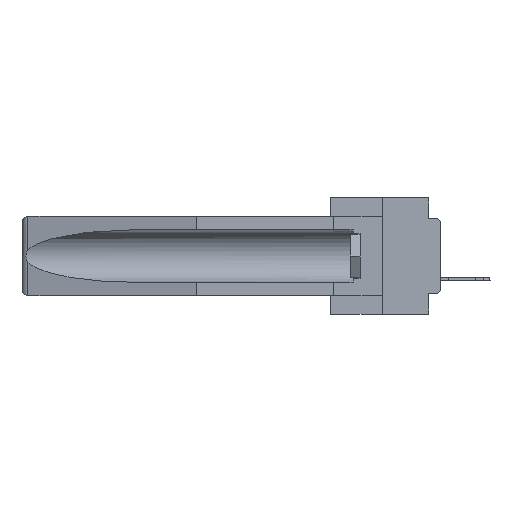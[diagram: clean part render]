
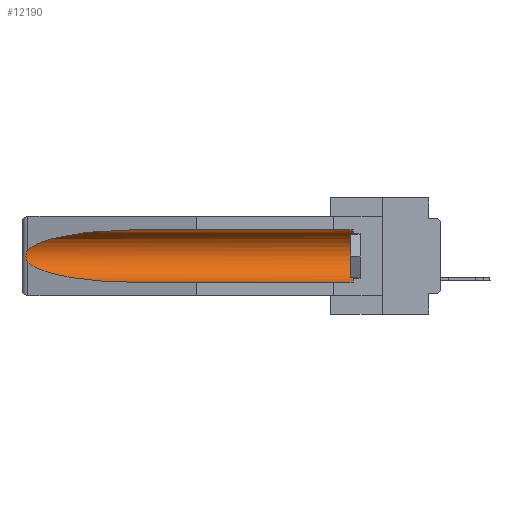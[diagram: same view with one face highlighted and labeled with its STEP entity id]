
A CAD part, left-side view. The second image highlights one B-rep face of the part: STEP entity #12190.
In plain terms, the highlighted cylindrical face has radius 2.857 mm (diameter 5.715 mm), a partial arc.
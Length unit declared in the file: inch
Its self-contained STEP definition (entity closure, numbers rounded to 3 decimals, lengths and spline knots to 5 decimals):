
#623 = CARTESIAN_POINT ( 'NONE',  ( 0.155, 1.07973, -0.059 ) ) ;
#852 = CARTESIAN_POINT ( 'NONE',  ( 0.26597, 1.5296, -0.19026 ) ) ;
#1108 = VERTEX_POINT ( 'NONE', #21107 ) ;
#1117 = EDGE_CURVE ( 'NONE', #18247, #1108, #5084, .T. ) ;
#1607 = DIRECTION ( 'NONE',  ( 0., 0., 1. ) ) ;
#1929 = CARTESIAN_POINT ( 'NONE',  ( 0.25451, 1.48313, -0.24835 ) ) ;
#3759 = ORIENTED_EDGE ( 'NONE', *, *, #10350, .T. ) ;
#4163 = CARTESIAN_POINT ( 'NONE',  ( 0.155, 1.07973, -0.284 ) ) ;
#5084 = CIRCLE ( 'NONE', #31580, 0.1125 ) ;
#5735 = VECTOR ( 'NONE', #5824, 39.37008 ) ;
#5824 = DIRECTION ( 'NONE',  ( 0., 1., 0. ) ) ;
#6933 = ORIENTED_EDGE ( 'NONE', *, *, #9786, .T. ) ;
#7885 = EDGE_CURVE ( 'NONE', #1108, #22006, #8084, .T. ) ;
#7907 = LINE ( 'NONE', #23471, #10756 ) ;
#7972 = EDGE_CURVE ( 'NONE', #18247, #27088, #7907, .T. ) ;
#8084 = LINE ( 'NONE', #13644, #5735 ) ;
#8950 = CARTESIAN_POINT ( 'NONE',  ( 0.26537, 1.52718, -0.19328 ) ) ;
#9365 = CARTESIAN_POINT ( 'NONE',  ( 0.21114, 1.30732, -0.284 ) ) ;
#9786 = EDGE_CURVE ( 'NONE', #22006, #15409, #31780, .T. ) ;
#9993 = VERTEX_POINT ( 'NONE', #33556 ) ;
#10173 = ORIENTED_EDGE ( 'NONE', *, *, #7885, .T. ) ;
#10350 = EDGE_CURVE ( 'NONE', #9993, #27088, #11531, .T. ) ;
#10549 = ORIENTED_EDGE ( 'NONE', *, *, #1117, .T. ) ;
#10756 = VECTOR ( 'NONE', #15705, 39.37008 ) ;
#11163 = CARTESIAN_POINT ( 'NONE',  ( 0.25451, 1.48313, -0.09465 ) ) ;
#11531 =( BOUNDED_CURVE ( )  B_SPLINE_CURVE ( 3, ( #27660, #1929, #9365, #4163 ),
 .UNSPECIFIED., .F., .F. ) 
 B_SPLINE_CURVE_WITH_KNOTS ( ( 4, 4 ),
 ( 0.1948, 1.5708 ),
 .UNSPECIFIED. ) 
 CURVE ( )  GEOMETRIC_REPRESENTATION_ITEM ( )  RATIONAL_B_SPLINE_CURVE ( ( 1., 0.848, 0.848, 1. ) ) 
 REPRESENTATION_ITEM ( '' )  );
#11672 = CARTESIAN_POINT ( 'NONE',  ( 0.26537, 1.52718, -0.14972 ) ) ;
#11909 = CARTESIAN_POINT ( 'NONE',  ( 0.26654, 1.53092, -0.15636 ) ) ;
#12190 = ADVANCED_FACE ( 'NONE', ( #33198 ), #25284, .F. ) ;
#12943 = ORIENTED_EDGE ( 'NONE', *, *, #7972, .F. ) ;
#13644 = CARTESIAN_POINT ( 'NONE',  ( 0.155, -0.30754, -0.059 ) ) ;
#13938 = CARTESIAN_POINT ( 'NONE',  ( 0.21114, 1.30732, -0.059 ) ) ;
#14508 = CARTESIAN_POINT ( 'NONE',  ( 0.26597, 1.52961, -0.15275 ) ) ;
#15085 = CARTESIAN_POINT ( 'NONE',  ( 0.26537, 1.52718, -0.14972 ) ) ;
#15409 = VERTEX_POINT ( 'NONE', #15085 ) ;
#15705 = DIRECTION ( 'NONE',  ( 0., 1., 0. ) ) ;
#18247 = VERTEX_POINT ( 'NONE', #25993 ) ;
#19043 = CARTESIAN_POINT ( 'NONE',  ( 0.155, 0.126, -0.1715 ) ) ;
#21107 = CARTESIAN_POINT ( 'NONE',  ( 0.155, 0.126, -0.059 ) ) ;
#22006 = VERTEX_POINT ( 'NONE', #32040 ) ;
#22587 = CARTESIAN_POINT ( 'NONE',  ( 0.2675, 1.53308, -0.16763 ) ) ;
#23471 = CARTESIAN_POINT ( 'NONE',  ( 0.155, -0.30754, -0.284 ) ) ;
#24680 = CARTESIAN_POINT ( 'NONE',  ( 0.26537, 1.52718, -0.14972 ) ) ;
#24832 = EDGE_CURVE ( 'NONE', #15409, #9993, #32712, .T. ) ;
#25284 = CYLINDRICAL_SURFACE ( 'NONE', #26852, 0.1125 ) ;
#25993 = CARTESIAN_POINT ( 'NONE',  ( 0.155, 0.126, -0.284 ) ) ;
#26802 = DIRECTION ( 'NONE',  ( 0., -1., 0. ) ) ;
#26852 = AXIS2_PLACEMENT_3D ( 'NONE', #30951, #28198, #1607 ) ;
#26955 = DIRECTION ( 'NONE',  ( 0., 0., 1. ) ) ;
#27088 = VERTEX_POINT ( 'NONE', #33019 ) ;
#27593 = CARTESIAN_POINT ( 'NONE',  ( 0.26655, 1.53094, -0.18657 ) ) ;
#27660 = CARTESIAN_POINT ( 'NONE',  ( 0.26537, 1.52718, -0.19328 ) ) ;
#27757 = CARTESIAN_POINT ( 'NONE',  ( 0.2673, 1.5327, -0.16383 ) ) ;
#28198 = DIRECTION ( 'NONE',  ( 0., 1., 0. ) ) ;
#29670 = CARTESIAN_POINT ( 'NONE',  ( 0.2673, 1.53269, -0.17917 ) ) ;
#29687 = ORIENTED_EDGE ( 'NONE', *, *, #24832, .T. ) ;
#30430 = EDGE_LOOP ( 'NONE', ( #6933, #29687, #3759, #12943, #10549, #10173 ) ) ;
#30951 = CARTESIAN_POINT ( 'NONE',  ( 0.155, -0.30754, -0.1715 ) ) ;
#31580 = AXIS2_PLACEMENT_3D ( 'NONE', #19043, #26802, #26955 ) ;
#31780 =( BOUNDED_CURVE ( )  B_SPLINE_CURVE ( 3, ( #623, #13938, #11163, #11672 ),
 .UNSPECIFIED., .F., .F. ) 
 B_SPLINE_CURVE_WITH_KNOTS ( ( 4, 4 ),
 ( 4.71239, 6.08839 ),
 .UNSPECIFIED. ) 
 CURVE ( )  GEOMETRIC_REPRESENTATION_ITEM ( )  RATIONAL_B_SPLINE_CURVE ( ( 1., 0.848, 0.848, 1. ) ) 
 REPRESENTATION_ITEM ( '' )  );
#32040 = CARTESIAN_POINT ( 'NONE',  ( 0.155, 1.07973, -0.059 ) ) ;
#32712 = B_SPLINE_CURVE_WITH_KNOTS ( 'NONE', 3,
 ( #24680, #14508, #11909, #27757, #22587, #33103, #29670, #27593, #852, #8950 ),
 .UNSPECIFIED., .F., .F.,
 ( 4, 2, 2, 2, 4 ),
 ( 0., 0.00029, 0.00058, 0.00087, 0.00117 ),
 .UNSPECIFIED. ) ;
#33019 = CARTESIAN_POINT ( 'NONE',  ( 0.155, 1.07973, -0.284 ) ) ;
#33103 = CARTESIAN_POINT ( 'NONE',  ( 0.2675, 1.53308, -0.17534 ) ) ;
#33198 = FACE_OUTER_BOUND ( 'NONE', #30430, .T. ) ;
#33556 = CARTESIAN_POINT ( 'NONE',  ( 0.26537, 1.52718, -0.19328 ) ) ;
